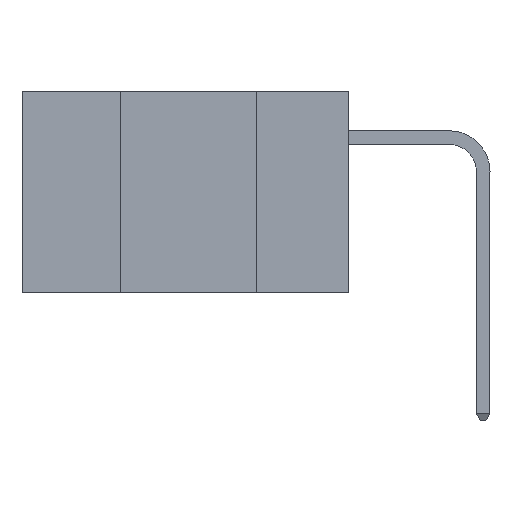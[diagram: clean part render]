
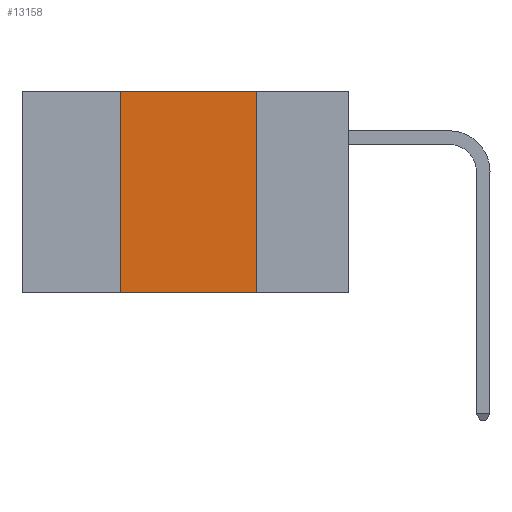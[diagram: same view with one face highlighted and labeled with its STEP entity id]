
A CAD part, left-side view. The second image highlights one B-rep face of the part: STEP entity #13158.
In plain terms, the highlighted planar face has unit normal (-1, 0, 0).
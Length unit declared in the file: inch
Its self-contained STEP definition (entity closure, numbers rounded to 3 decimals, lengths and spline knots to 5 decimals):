
#1019 = CARTESIAN_POINT ( 'NONE',  ( 0., 0.6, 0. ) ) ;
#1340 = VECTOR ( 'NONE', #13021, 39.37008 ) ;
#1355 = VERTEX_POINT ( 'NONE', #8775 ) ;
#1457 = CARTESIAN_POINT ( 'NONE',  ( 0., 0.42, 0. ) ) ;
#2124 = LINE ( 'NONE', #8936, #8479 ) ;
#2316 = EDGE_CURVE ( 'NONE', #12384, #1355, #7136, .T. ) ;
#3124 = LINE ( 'NONE', #6858, #9444 ) ;
#3946 = ORIENTED_EDGE ( 'NONE', *, *, #2316, .F. ) ;
#4190 = ORIENTED_EDGE ( 'NONE', *, *, #5135, .F. ) ;
#5135 = EDGE_CURVE ( 'NONE', #1355, #11549, #2124, .T. ) ;
#5929 = EDGE_CURVE ( 'NONE', #12855, #12384, #6426, .T. ) ;
#6202 = CARTESIAN_POINT ( 'NONE',  ( 0., 0.42, -0.37 ) ) ;
#6418 = VECTOR ( 'NONE', #13897, 39.37008 ) ;
#6426 = LINE ( 'NONE', #1457, #1340 ) ;
#6858 = CARTESIAN_POINT ( 'NONE',  ( 0., 0.6, -0.37 ) ) ;
#7136 = LINE ( 'NONE', #1019, #6418 ) ;
#7790 = DIRECTION ( 'NONE',  ( 0., 0., -1. ) ) ;
#8013 = EDGE_CURVE ( 'NONE', #12855, #11549, #3124, .T. ) ;
#8276 = ORIENTED_EDGE ( 'NONE', *, *, #8013, .T. ) ;
#8303 = EDGE_LOOP ( 'NONE', ( #4190, #3946, #10466, #8276 ) ) ;
#8323 = CARTESIAN_POINT ( 'NONE',  ( 0., 0.17, -0.37 ) ) ;
#8479 = VECTOR ( 'NONE', #7790, 39.37008 ) ;
#8601 = FACE_OUTER_BOUND ( 'NONE', #8303, .T. ) ;
#8775 = CARTESIAN_POINT ( 'NONE',  ( 0., 0.17, 0. ) ) ;
#8936 = CARTESIAN_POINT ( 'NONE',  ( 0., 0.17, 0. ) ) ;
#9444 = VECTOR ( 'NONE', #12732, 39.37008 ) ;
#9867 = PLANE ( 'NONE',  #14435 ) ;
#9925 = CARTESIAN_POINT ( 'NONE',  ( 0., 0.6, 0. ) ) ;
#10466 = ORIENTED_EDGE ( 'NONE', *, *, #5929, .F. ) ;
#10835 = CARTESIAN_POINT ( 'NONE',  ( 0., 0.42, 0. ) ) ;
#11021 = DIRECTION ( 'NONE',  ( 1., 0., 0. ) ) ;
#11549 = VERTEX_POINT ( 'NONE', #8323 ) ;
#12384 = VERTEX_POINT ( 'NONE', #10835 ) ;
#12400 = DIRECTION ( 'NONE',  ( 0., 0., -1. ) ) ;
#12732 = DIRECTION ( 'NONE',  ( 0., -1., 0. ) ) ;
#12855 = VERTEX_POINT ( 'NONE', #6202 ) ;
#13021 = DIRECTION ( 'NONE',  ( 0., 0., 1. ) ) ;
#13158 = ADVANCED_FACE ( 'NONE', ( #8601 ), #9867, .F. ) ;
#13897 = DIRECTION ( 'NONE',  ( 0., -1., 0. ) ) ;
#14435 = AXIS2_PLACEMENT_3D ( 'NONE', #9925, #11021, #12400 ) ;
